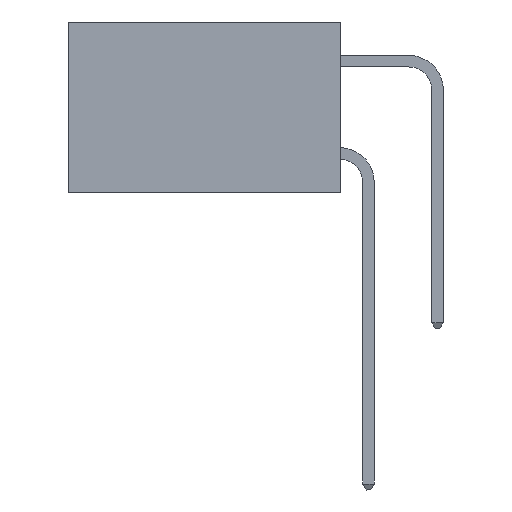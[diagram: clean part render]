
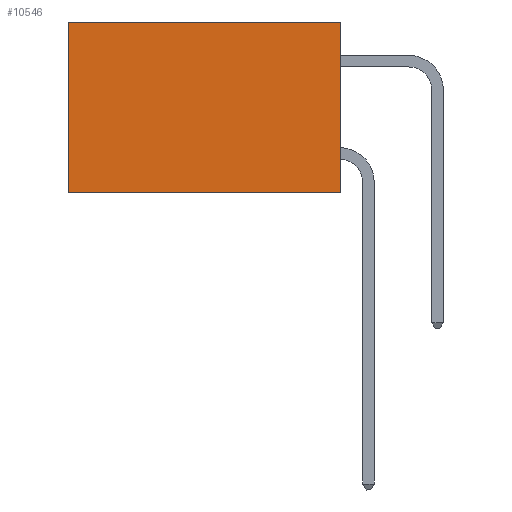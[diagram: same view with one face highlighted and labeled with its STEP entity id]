
A CAD part, left-side view. The second image highlights one B-rep face of the part: STEP entity #10546.
In plain terms, the highlighted planar face has unit normal (-1, 0, 0).
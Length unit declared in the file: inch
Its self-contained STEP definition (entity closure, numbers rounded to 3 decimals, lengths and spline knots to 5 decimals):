
#192 = LINE ( 'NONE', #10796, #5787 ) ;
#303 = EDGE_CURVE ( 'NONE', #8949, #1582, #192, .T. ) ;
#332 = CARTESIAN_POINT ( 'NONE',  ( 0.277, 0.59, -0.37 ) ) ;
#897 = PLANE ( 'NONE',  #6788 ) ;
#1582 = VERTEX_POINT ( 'NONE', #332 ) ;
#2015 = DIRECTION ( 'NONE',  ( 1., 0., 0. ) ) ;
#2167 = EDGE_CURVE ( 'NONE', #12482, #3063, #11825, .T. ) ;
#3054 = VECTOR ( 'NONE', #13640, 39.37008 ) ;
#3063 = VERTEX_POINT ( 'NONE', #10629 ) ;
#3530 = EDGE_CURVE ( 'NONE', #12482, #8949, #11133, .T. ) ;
#4259 = CARTESIAN_POINT ( 'NONE',  ( 0.277, 0., 0. ) ) ;
#4349 = DIRECTION ( 'NONE',  ( 0., 1., 0. ) ) ;
#4711 = LINE ( 'NONE', #6105, #7689 ) ;
#5312 = VECTOR ( 'NONE', #4349, 39.37008 ) ;
#5787 = VECTOR ( 'NONE', #10880, 39.37008 ) ;
#5902 = ORIENTED_EDGE ( 'NONE', *, *, #303, .T. ) ;
#6105 = CARTESIAN_POINT ( 'NONE',  ( 0.277, 0., -0.37 ) ) ;
#6788 = AXIS2_PLACEMENT_3D ( 'NONE', #8673, #2015, #9786 ) ;
#7235 = DIRECTION ( 'NONE',  ( 0., 1., 0. ) ) ;
#7656 = CARTESIAN_POINT ( 'NONE',  ( 0.277, 0., 0. ) ) ;
#7689 = VECTOR ( 'NONE', #7235, 39.37008 ) ;
#8673 = CARTESIAN_POINT ( 'NONE',  ( 0.277, 0., -0.37 ) ) ;
#8874 = EDGE_CURVE ( 'NONE', #3063, #1582, #4711, .T. ) ;
#8949 = VERTEX_POINT ( 'NONE', #10554 ) ;
#9786 = DIRECTION ( 'NONE',  ( 0., 0., -1. ) ) ;
#10546 = ADVANCED_FACE ( 'NONE', ( #13601 ), #897, .F. ) ;
#10554 = CARTESIAN_POINT ( 'NONE',  ( 0.277, 0.59, 0. ) ) ;
#10629 = CARTESIAN_POINT ( 'NONE',  ( 0.277, 0., -0.37 ) ) ;
#10796 = CARTESIAN_POINT ( 'NONE',  ( 0.277, 0.59, -0.37 ) ) ;
#10864 = EDGE_LOOP ( 'NONE', ( #5902, #13975, #13194, #13354 ) ) ;
#10880 = DIRECTION ( 'NONE',  ( 0., 0., -1. ) ) ;
#11133 = LINE ( 'NONE', #4259, #5312 ) ;
#11825 = LINE ( 'NONE', #13869, #3054 ) ;
#12482 = VERTEX_POINT ( 'NONE', #7656 ) ;
#13194 = ORIENTED_EDGE ( 'NONE', *, *, #2167, .F. ) ;
#13354 = ORIENTED_EDGE ( 'NONE', *, *, #3530, .T. ) ;
#13601 = FACE_OUTER_BOUND ( 'NONE', #10864, .T. ) ;
#13640 = DIRECTION ( 'NONE',  ( 0., 0., -1. ) ) ;
#13869 = CARTESIAN_POINT ( 'NONE',  ( 0.277, 0., -0.37 ) ) ;
#13975 = ORIENTED_EDGE ( 'NONE', *, *, #8874, .F. ) ;
